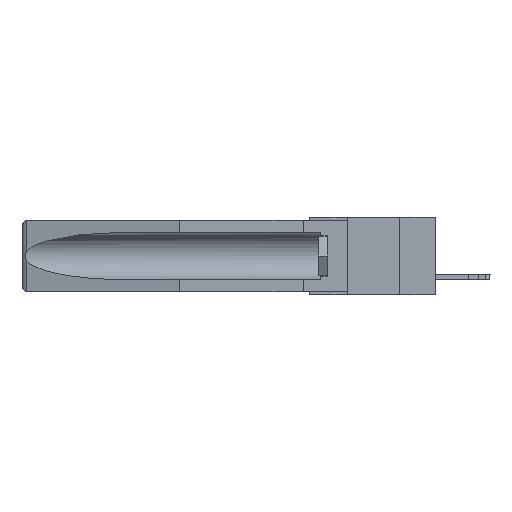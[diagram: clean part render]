
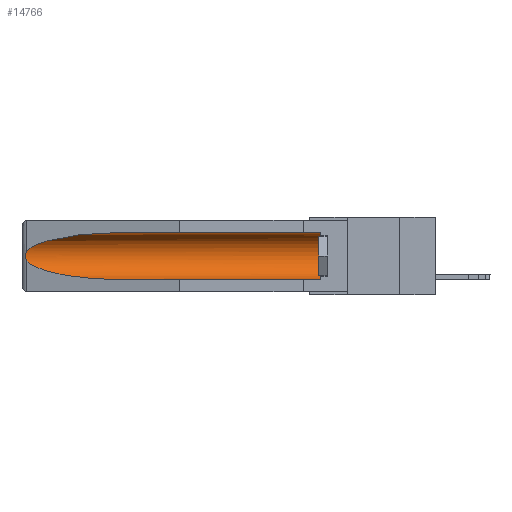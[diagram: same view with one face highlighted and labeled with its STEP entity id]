
A CAD part, left-side view. The second image highlights one B-rep face of the part: STEP entity #14766.
In plain terms, the highlighted cylindrical face has radius 2.857 mm (diameter 5.715 mm), a partial arc.
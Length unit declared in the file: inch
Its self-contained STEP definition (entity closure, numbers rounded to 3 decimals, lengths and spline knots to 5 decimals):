
#87 = VERTEX_POINT ( 'NONE', #8727 ) ;
#1263 = VECTOR ( 'NONE', #20111, 39.37008 ) ;
#1435 = CARTESIAN_POINT ( 'NONE',  ( 0.2673, 1.53269, -0.17917 ) ) ;
#1617 = EDGE_CURVE ( 'NONE', #87, #18779, #6214, .T. ) ;
#2248 = CARTESIAN_POINT ( 'NONE',  ( 0.155, 0.126, -0.284 ) ) ;
#2731 = CARTESIAN_POINT ( 'NONE',  ( 0.155, 0.126, -0.1715 ) ) ;
#3194 = CARTESIAN_POINT ( 'NONE',  ( 0.26537, 1.52718, -0.19328 ) ) ;
#3567 = CARTESIAN_POINT ( 'NONE',  ( 0.155, 1.07973, -0.059 ) ) ;
#3792 = DIRECTION ( 'NONE',  ( 0., 0., 1. ) ) ;
#4315 =( BOUNDED_CURVE ( )  B_SPLINE_CURVE ( 3, ( #18295, #24470, #12665, #6351 ),
 .UNSPECIFIED., .F., .F. ) 
 B_SPLINE_CURVE_WITH_KNOTS ( ( 4, 4 ),
 ( 4.71239, 6.08839 ),
 .UNSPECIFIED. ) 
 CURVE ( )  GEOMETRIC_REPRESENTATION_ITEM ( )  RATIONAL_B_SPLINE_CURVE ( ( 1., 0.848, 0.848, 1. ) ) 
 REPRESENTATION_ITEM ( '' )  );
#5120 = CARTESIAN_POINT ( 'NONE',  ( 0.26537, 1.52718, -0.19328 ) ) ;
#5402 = CARTESIAN_POINT ( 'NONE',  ( 0.26537, 1.52718, -0.14972 ) ) ;
#6214 = B_SPLINE_CURVE_WITH_KNOTS ( 'NONE', 3,
 ( #5402, #19629, #9314, #23241, #11346, #17314, #1435, #11434, #25326, #13447 ),
 .UNSPECIFIED., .F., .F.,
 ( 4, 2, 2, 2, 4 ),
 ( 0., 0.00029, 0.00058, 0.00087, 0.00117 ),
 .UNSPECIFIED. ) ;
#6351 = CARTESIAN_POINT ( 'NONE',  ( 0.26537, 1.52718, -0.14972 ) ) ;
#7133 = LINE ( 'NONE', #23645, #1263 ) ;
#8115 = EDGE_CURVE ( 'NONE', #18779, #16964, #13599, .T. ) ;
#8335 = CYLINDRICAL_SURFACE ( 'NONE', #24913, 0.1125 ) ;
#8651 = FACE_OUTER_BOUND ( 'NONE', #15226, .T. ) ;
#8679 = EDGE_CURVE ( 'NONE', #25402, #87, #4315, .T. ) ;
#8727 = CARTESIAN_POINT ( 'NONE',  ( 0.26537, 1.52718, -0.14972 ) ) ;
#9185 = CARTESIAN_POINT ( 'NONE',  ( 0.21114, 1.30732, -0.284 ) ) ;
#9314 = CARTESIAN_POINT ( 'NONE',  ( 0.26654, 1.53092, -0.15636 ) ) ;
#10378 = EDGE_CURVE ( 'NONE', #24298, #25402, #7133, .T. ) ;
#10816 = ORIENTED_EDGE ( 'NONE', *, *, #8115, .T. ) ;
#11220 = CARTESIAN_POINT ( 'NONE',  ( 0.155, 1.07973, -0.284 ) ) ;
#11346 = CARTESIAN_POINT ( 'NONE',  ( 0.2675, 1.53308, -0.16763 ) ) ;
#11408 = EDGE_CURVE ( 'NONE', #16338, #16964, #15782, .T. ) ;
#11434 = CARTESIAN_POINT ( 'NONE',  ( 0.26655, 1.53094, -0.18657 ) ) ;
#12095 = ORIENTED_EDGE ( 'NONE', *, *, #20475, .T. ) ;
#12141 = ORIENTED_EDGE ( 'NONE', *, *, #11408, .F. ) ;
#12665 = CARTESIAN_POINT ( 'NONE',  ( 0.25451, 1.48313, -0.09465 ) ) ;
#13447 = CARTESIAN_POINT ( 'NONE',  ( 0.26537, 1.52718, -0.19328 ) ) ;
#13599 =( BOUNDED_CURVE ( )  B_SPLINE_CURVE ( 3, ( #3194, #19243, #9185, #11220 ),
 .UNSPECIFIED., .F., .F. ) 
 B_SPLINE_CURVE_WITH_KNOTS ( ( 4, 4 ),
 ( 0.1948, 1.5708 ),
 .UNSPECIFIED. ) 
 CURVE ( )  GEOMETRIC_REPRESENTATION_ITEM ( )  RATIONAL_B_SPLINE_CURVE ( ( 1., 0.848, 0.848, 1. ) ) 
 REPRESENTATION_ITEM ( '' )  );
#14766 = ADVANCED_FACE ( 'NONE', ( #8651 ), #8335, .F. ) ;
#15226 = EDGE_LOOP ( 'NONE', ( #25665, #22833, #10816, #12141, #12095, #20872 ) ) ;
#15661 = CARTESIAN_POINT ( 'NONE',  ( 0.155, 1.07973, -0.284 ) ) ;
#15712 = DIRECTION ( 'NONE',  ( 0., 1., 0. ) ) ;
#15782 = LINE ( 'NONE', #24276, #16082 ) ;
#16082 = VECTOR ( 'NONE', #24360, 39.37008 ) ;
#16338 = VERTEX_POINT ( 'NONE', #2248 ) ;
#16964 = VERTEX_POINT ( 'NONE', #15661 ) ;
#17314 = CARTESIAN_POINT ( 'NONE',  ( 0.2675, 1.53308, -0.17534 ) ) ;
#18295 = CARTESIAN_POINT ( 'NONE',  ( 0.155, 1.07973, -0.059 ) ) ;
#18779 = VERTEX_POINT ( 'NONE', #5120 ) ;
#19243 = CARTESIAN_POINT ( 'NONE',  ( 0.25451, 1.48313, -0.24835 ) ) ;
#19629 = CARTESIAN_POINT ( 'NONE',  ( 0.26597, 1.52961, -0.15275 ) ) ;
#20111 = DIRECTION ( 'NONE',  ( 0., 1., 0. ) ) ;
#20475 = EDGE_CURVE ( 'NONE', #16338, #24298, #21930, .T. ) ;
#20872 = ORIENTED_EDGE ( 'NONE', *, *, #10378, .T. ) ;
#21930 = CIRCLE ( 'NONE', #25307, 0.1125 ) ;
#22646 = DIRECTION ( 'NONE',  ( 0., -1., 0. ) ) ;
#22756 = CARTESIAN_POINT ( 'NONE',  ( 0.155, 0.126, -0.059 ) ) ;
#22833 = ORIENTED_EDGE ( 'NONE', *, *, #1617, .T. ) ;
#22893 = DIRECTION ( 'NONE',  ( 0., 0., 1. ) ) ;
#23241 = CARTESIAN_POINT ( 'NONE',  ( 0.2673, 1.5327, -0.16383 ) ) ;
#23645 = CARTESIAN_POINT ( 'NONE',  ( 0.155, -0.30754, -0.059 ) ) ;
#23652 = CARTESIAN_POINT ( 'NONE',  ( 0.155, -0.30754, -0.1715 ) ) ;
#24276 = CARTESIAN_POINT ( 'NONE',  ( 0.155, -0.30754, -0.284 ) ) ;
#24298 = VERTEX_POINT ( 'NONE', #22756 ) ;
#24360 = DIRECTION ( 'NONE',  ( 0., 1., 0. ) ) ;
#24470 = CARTESIAN_POINT ( 'NONE',  ( 0.21114, 1.30732, -0.059 ) ) ;
#24913 = AXIS2_PLACEMENT_3D ( 'NONE', #23652, #15712, #3792 ) ;
#25307 = AXIS2_PLACEMENT_3D ( 'NONE', #2731, #22646, #22893 ) ;
#25326 = CARTESIAN_POINT ( 'NONE',  ( 0.26597, 1.5296, -0.19026 ) ) ;
#25402 = VERTEX_POINT ( 'NONE', #3567 ) ;
#25665 = ORIENTED_EDGE ( 'NONE', *, *, #8679, .T. ) ;
